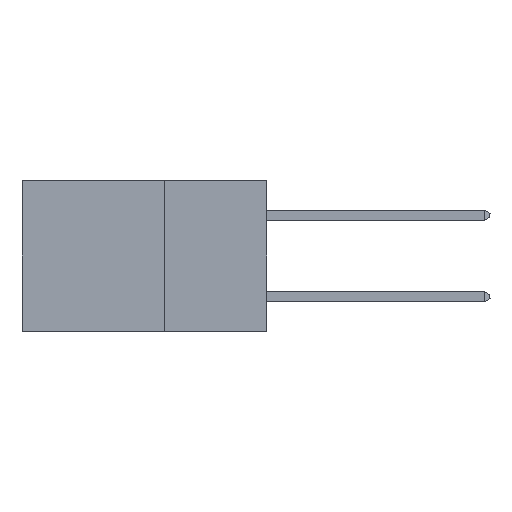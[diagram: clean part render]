
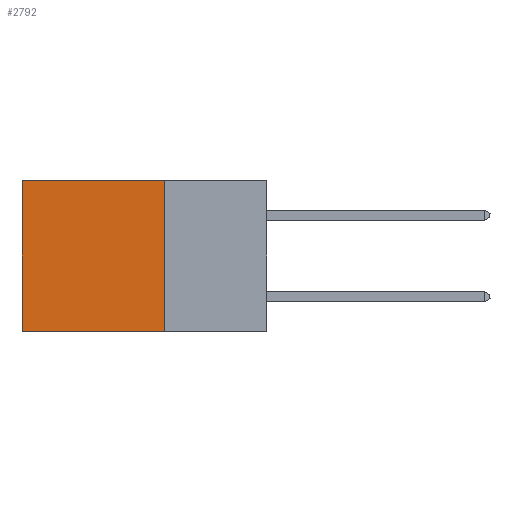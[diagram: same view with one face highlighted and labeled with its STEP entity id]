
A CAD part, left-side view. The second image highlights one B-rep face of the part: STEP entity #2792.
In plain terms, the highlighted planar face has unit normal (-1, 0, 0).
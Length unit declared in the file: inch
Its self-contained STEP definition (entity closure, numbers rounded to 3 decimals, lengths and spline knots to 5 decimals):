
#414 = FACE_OUTER_BOUND ( 'NONE', #9150, .T. ) ;
#2542 = PLANE ( 'NONE',  #18699 ) ;
#2570 = EDGE_CURVE ( 'NONE', #15341, #15558, #22393, .T. ) ;
#2792 = ADVANCED_FACE ( 'NONE', ( #414 ), #2542, .F. ) ;
#3791 = EDGE_CURVE ( 'NONE', #18480, #15341, #14120, .T. ) ;
#3925 = VECTOR ( 'NONE', #9954, 39.37008 ) ;
#4339 = ORIENTED_EDGE ( 'NONE', *, *, #3791, .T. ) ;
#4529 = ORIENTED_EDGE ( 'NONE', *, *, #18095, .F. ) ;
#5975 = ORIENTED_EDGE ( 'NONE', *, *, #2570, .T. ) ;
#6634 = DIRECTION ( 'NONE',  ( 0., 0., -1. ) ) ;
#8326 = ORIENTED_EDGE ( 'NONE', *, *, #10735, .F. ) ;
#9150 = EDGE_LOOP ( 'NONE', ( #5975, #4529, #8326, #4339 ) ) ;
#9923 = CARTESIAN_POINT ( 'NONE',  ( 0.2875, 0.6, 0. ) ) ;
#9954 = DIRECTION ( 'NONE',  ( 0., 1., 0. ) ) ;
#10696 = DIRECTION ( 'NONE',  ( 0., 1., 0. ) ) ;
#10735 = EDGE_CURVE ( 'NONE', #18480, #22946, #15708, .T. ) ;
#14120 = LINE ( 'NONE', #20106, #3925 ) ;
#15341 = VERTEX_POINT ( 'NONE', #22103 ) ;
#15558 = VERTEX_POINT ( 'NONE', #16710 ) ;
#15708 = LINE ( 'NONE', #16439, #20436 ) ;
#16439 = CARTESIAN_POINT ( 'NONE',  ( 0.2875, 0.25, 0. ) ) ;
#16710 = CARTESIAN_POINT ( 'NONE',  ( 0.2875, 0.6, -0.37 ) ) ;
#16779 = CARTESIAN_POINT ( 'NONE',  ( 0.2875, 0.25, 0. ) ) ;
#16921 = LINE ( 'NONE', #20849, #21667 ) ;
#16974 = CARTESIAN_POINT ( 'NONE',  ( 0.2875, 0.25, 0. ) ) ;
#18095 = EDGE_CURVE ( 'NONE', #22946, #15558, #16921, .T. ) ;
#18134 = DIRECTION ( 'NONE',  ( 0., 0., -1. ) ) ;
#18480 = VERTEX_POINT ( 'NONE', #16974 ) ;
#18699 = AXIS2_PLACEMENT_3D ( 'NONE', #16779, #18837, #6634 ) ;
#18837 = DIRECTION ( 'NONE',  ( 1., 0., 0. ) ) ;
#18839 = CARTESIAN_POINT ( 'NONE',  ( 0.2875, 0.25, -0.37 ) ) ;
#20106 = CARTESIAN_POINT ( 'NONE',  ( 0.2875, 0.25, 0. ) ) ;
#20436 = VECTOR ( 'NONE', #20504, 39.37008 ) ;
#20504 = DIRECTION ( 'NONE',  ( 0., 0., -1. ) ) ;
#20849 = CARTESIAN_POINT ( 'NONE',  ( 0.2875, 0.25, -0.37 ) ) ;
#21667 = VECTOR ( 'NONE', #10696, 39.37008 ) ;
#21760 = VECTOR ( 'NONE', #18134, 39.37008 ) ;
#22103 = CARTESIAN_POINT ( 'NONE',  ( 0.2875, 0.6, 0. ) ) ;
#22393 = LINE ( 'NONE', #9923, #21760 ) ;
#22946 = VERTEX_POINT ( 'NONE', #18839 ) ;
